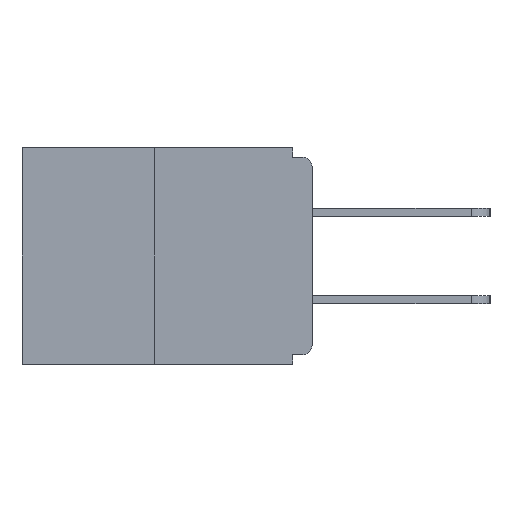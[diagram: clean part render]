
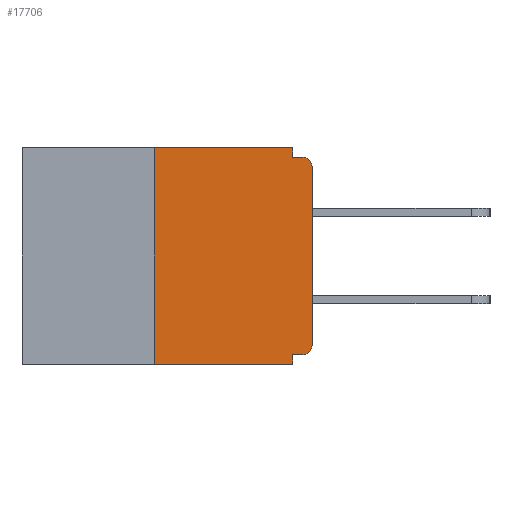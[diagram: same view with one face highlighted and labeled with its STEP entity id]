
A CAD part, left-side view. The second image highlights one B-rep face of the part: STEP entity #17706.
In plain terms, the highlighted planar face has unit normal (-1, 0, 0).
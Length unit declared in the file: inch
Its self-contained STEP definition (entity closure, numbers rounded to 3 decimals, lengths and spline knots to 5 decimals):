
#8 = LINE ( 'NONE', #19246, #6103 ) ;
#179 = CARTESIAN_POINT ( 'NONE',  ( 0., 0.015, -0.313 ) ) ;
#351 = VERTEX_POINT ( 'NONE', #14701 ) ;
#451 = EDGE_CURVE ( 'NONE', #17365, #647, #9772, .T. ) ;
#647 = VERTEX_POINT ( 'NONE', #4728 ) ;
#786 = ORIENTED_EDGE ( 'NONE', *, *, #3188, .T. ) ;
#1545 = AXIS2_PLACEMENT_3D ( 'NONE', #179, #18692, #12447 ) ;
#1617 = VECTOR ( 'NONE', #16616, 39.37008 ) ;
#1840 = ORIENTED_EDGE ( 'NONE', *, *, #451, .F. ) ;
#1945 = VECTOR ( 'NONE', #18155, 39.37008 ) ;
#1963 = VERTEX_POINT ( 'NONE', #18316 ) ;
#2064 = CARTESIAN_POINT ( 'NONE',  ( 0., 0.015, -0.328 ) ) ;
#2145 = VECTOR ( 'NONE', #19223, 39.37008 ) ;
#3031 = LINE ( 'NONE', #9881, #6673 ) ;
#3153 = ORIENTED_EDGE ( 'NONE', *, *, #18493, .T. ) ;
#3188 = EDGE_CURVE ( 'NONE', #10440, #18833, #16629, .T. ) ;
#3402 = VERTEX_POINT ( 'NONE', #2064 ) ;
#3559 = CARTESIAN_POINT ( 'NONE',  ( 0., 0.031, 0. ) ) ;
#3675 = LINE ( 'NONE', #12361, #15902 ) ;
#3942 = CARTESIAN_POINT ( 'NONE',  ( 0., 0., -0.03 ) ) ;
#4117 = EDGE_CURVE ( 'NONE', #3402, #17746, #12576, .T. ) ;
#4728 = CARTESIAN_POINT ( 'NONE',  ( 0., 0.031, -0.343 ) ) ;
#4951 = DIRECTION ( 'NONE',  ( 0., -1., 0. ) ) ;
#5057 = CARTESIAN_POINT ( 'NONE',  ( 0., 0.015, -0.03 ) ) ;
#5554 = DIRECTION ( 'NONE',  ( 0., -1., 0. ) ) ;
#5794 = LINE ( 'NONE', #14981, #18748 ) ;
#5801 = EDGE_CURVE ( 'NONE', #351, #16977, #8, .T. ) ;
#5882 = ORIENTED_EDGE ( 'NONE', *, *, #16561, .F. ) ;
#5894 = EDGE_CURVE ( 'NONE', #3402, #17365, #14218, .T. ) ;
#5961 = ORIENTED_EDGE ( 'NONE', *, *, #6934, .F. ) ;
#6103 = VECTOR ( 'NONE', #5554, 39.37008 ) ;
#6673 = VECTOR ( 'NONE', #12726, 39.37008 ) ;
#6934 = EDGE_CURVE ( 'NONE', #1963, #351, #19021, .T. ) ;
#7136 = EDGE_LOOP ( 'NONE', ( #12812, #5961, #8432, #1840, #19835, #16053, #3153, #786, #16631, #5882 ) ) ;
#7824 = AXIS2_PLACEMENT_3D ( 'NONE', #18663, #10999, #12550 ) ;
#7874 = AXIS2_PLACEMENT_3D ( 'NONE', #5057, #17118, #9489 ) ;
#7898 = LINE ( 'NONE', #14846, #1617 ) ;
#8079 = EDGE_CURVE ( 'NONE', #13278, #18833, #7898, .T. ) ;
#8432 = ORIENTED_EDGE ( 'NONE', *, *, #12350, .T. ) ;
#8526 = CARTESIAN_POINT ( 'NONE',  ( 0., 0.031, -0.015 ) ) ;
#8991 = DIRECTION ( 'NONE',  ( 0., 0., 1. ) ) ;
#9489 = DIRECTION ( 'NONE',  ( 0., 0., -1. ) ) ;
#9772 = LINE ( 'NONE', #11863, #10755 ) ;
#9881 = CARTESIAN_POINT ( 'NONE',  ( 0., 0.031, 0. ) ) ;
#10440 = VERTEX_POINT ( 'NONE', #3942 ) ;
#10621 = FACE_OUTER_BOUND ( 'NONE', #7136, .T. ) ;
#10727 = CARTESIAN_POINT ( 'NONE',  ( 0., 0.25, 0. ) ) ;
#10755 = VECTOR ( 'NONE', #14824, 39.37008 ) ;
#10847 = CARTESIAN_POINT ( 'NONE',  ( 0., 0., -0.313 ) ) ;
#10999 = DIRECTION ( 'NONE',  ( 1., 0., 0. ) ) ;
#11041 = PLANE ( 'NONE',  #7824 ) ;
#11863 = CARTESIAN_POINT ( 'NONE',  ( 0., 0.031, -0.343 ) ) ;
#12350 = EDGE_CURVE ( 'NONE', #1963, #647, #3675, .T. ) ;
#12361 = CARTESIAN_POINT ( 'NONE',  ( 0., 0.46, -0.343 ) ) ;
#12447 = DIRECTION ( 'NONE',  ( 0., 0., -1. ) ) ;
#12550 = DIRECTION ( 'NONE',  ( 0., 0., -1. ) ) ;
#12576 = CIRCLE ( 'NONE', #1545, 0.015 ) ;
#12726 = DIRECTION ( 'NONE',  ( 0., 0., -1. ) ) ;
#12812 = ORIENTED_EDGE ( 'NONE', *, *, #5801, .F. ) ;
#12866 = CARTESIAN_POINT ( 'NONE',  ( 0., 0.015, -0.015 ) ) ;
#12879 = CARTESIAN_POINT ( 'NONE',  ( 0., 0.031, -0.328 ) ) ;
#13278 = VERTEX_POINT ( 'NONE', #8526 ) ;
#14218 = LINE ( 'NONE', #14951, #1945 ) ;
#14701 = CARTESIAN_POINT ( 'NONE',  ( 0., 0.25, 0. ) ) ;
#14824 = DIRECTION ( 'NONE',  ( 0., 0., -1. ) ) ;
#14846 = CARTESIAN_POINT ( 'NONE',  ( 0., 0., -0.015 ) ) ;
#14951 = CARTESIAN_POINT ( 'NONE',  ( 0., 0., -0.328 ) ) ;
#14981 = CARTESIAN_POINT ( 'NONE',  ( 0., 0., 0. ) ) ;
#15902 = VECTOR ( 'NONE', #4951, 39.37008 ) ;
#16053 = ORIENTED_EDGE ( 'NONE', *, *, #4117, .T. ) ;
#16561 = EDGE_CURVE ( 'NONE', #16977, #13278, #3031, .T. ) ;
#16616 = DIRECTION ( 'NONE',  ( 0., -1., 0. ) ) ;
#16629 = CIRCLE ( 'NONE', #7874, 0.015 ) ;
#16631 = ORIENTED_EDGE ( 'NONE', *, *, #8079, .F. ) ;
#16977 = VERTEX_POINT ( 'NONE', #3559 ) ;
#17118 = DIRECTION ( 'NONE',  ( -1., 0., 0. ) ) ;
#17365 = VERTEX_POINT ( 'NONE', #12879 ) ;
#17706 = ADVANCED_FACE ( 'NONE', ( #10621 ), #11041, .F. ) ;
#17746 = VERTEX_POINT ( 'NONE', #10847 ) ;
#18155 = DIRECTION ( 'NONE',  ( 0., 1., 0. ) ) ;
#18316 = CARTESIAN_POINT ( 'NONE',  ( 0., 0.25, -0.343 ) ) ;
#18493 = EDGE_CURVE ( 'NONE', #17746, #10440, #5794, .T. ) ;
#18663 = CARTESIAN_POINT ( 'NONE',  ( 0., 0.46, 0. ) ) ;
#18692 = DIRECTION ( 'NONE',  ( -1., 0., 0. ) ) ;
#18748 = VECTOR ( 'NONE', #8991, 39.37008 ) ;
#18833 = VERTEX_POINT ( 'NONE', #12866 ) ;
#19021 = LINE ( 'NONE', #10727, #2145 ) ;
#19223 = DIRECTION ( 'NONE',  ( 0., 0., 1. ) ) ;
#19246 = CARTESIAN_POINT ( 'NONE',  ( 0., 0.46, 0. ) ) ;
#19835 = ORIENTED_EDGE ( 'NONE', *, *, #5894, .F. ) ;
